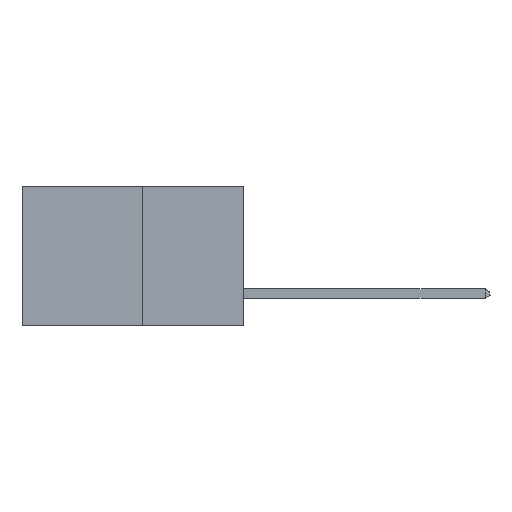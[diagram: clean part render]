
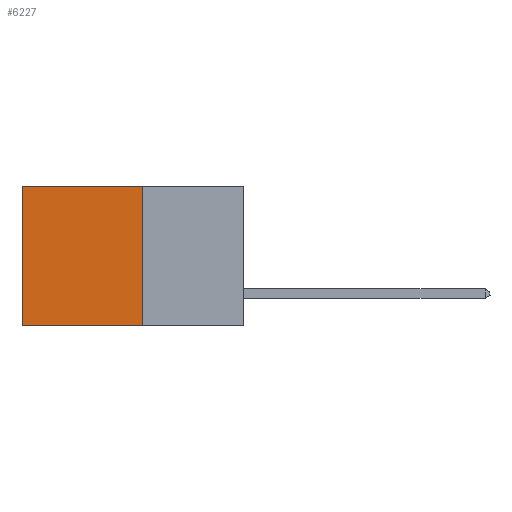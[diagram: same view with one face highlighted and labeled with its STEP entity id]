
A CAD part, left-side view. The second image highlights one B-rep face of the part: STEP entity #6227.
In plain terms, the highlighted planar face has unit normal (-1, 0, 0).
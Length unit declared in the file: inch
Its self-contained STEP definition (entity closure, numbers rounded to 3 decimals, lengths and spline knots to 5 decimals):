
#29 = LINE ( 'NONE', #17643, #5510 ) ;
#1567 = FACE_OUTER_BOUND ( 'NONE', #23449, .T. ) ;
#1588 = ORIENTED_EDGE ( 'NONE', *, *, #8246, .T. ) ;
#4733 = CARTESIAN_POINT ( 'NONE',  ( 0.277, 0.27, 0. ) ) ;
#4839 = CARTESIAN_POINT ( 'NONE',  ( 0.277, 0.59, -0.37 ) ) ;
#5190 = LINE ( 'NONE', #4733, #28686 ) ;
#5510 = VECTOR ( 'NONE', #18485, 39.37008 ) ;
#5772 = DIRECTION ( 'NONE',  ( 0., 1., 0. ) ) ;
#6227 = ADVANCED_FACE ( 'NONE', ( #1567 ), #15031, .F. ) ;
#8246 = EDGE_CURVE ( 'NONE', #19467, #26745, #29, .T. ) ;
#9093 = EDGE_CURVE ( 'NONE', #21050, #10679, #17947, .T. ) ;
#9815 = CARTESIAN_POINT ( 'NONE',  ( 0.277, 0.27, 0. ) ) ;
#10679 = VERTEX_POINT ( 'NONE', #17119 ) ;
#11189 = CARTESIAN_POINT ( 'NONE',  ( 0.277, 0.27, -0.37 ) ) ;
#11669 = VECTOR ( 'NONE', #21087, 39.37008 ) ;
#11834 = LINE ( 'NONE', #11189, #29878 ) ;
#12332 = ORIENTED_EDGE ( 'NONE', *, *, #19632, .F. ) ;
#15031 = PLANE ( 'NONE',  #21664 ) ;
#15071 = DIRECTION ( 'NONE',  ( 0., 0., -1. ) ) ;
#15459 = ORIENTED_EDGE ( 'NONE', *, *, #16561, .T. ) ;
#16561 = EDGE_CURVE ( 'NONE', #21050, #19467, #5190, .T. ) ;
#16855 = ORIENTED_EDGE ( 'NONE', *, *, #9093, .F. ) ;
#17119 = CARTESIAN_POINT ( 'NONE',  ( 0.277, 0.27, -0.37 ) ) ;
#17614 = DIRECTION ( 'NONE',  ( 1., 0., 0. ) ) ;
#17643 = CARTESIAN_POINT ( 'NONE',  ( 0.277, 0.59, -0.37 ) ) ;
#17775 = CARTESIAN_POINT ( 'NONE',  ( 0.277, 0.59, 0. ) ) ;
#17947 = LINE ( 'NONE', #30045, #11669 ) ;
#18485 = DIRECTION ( 'NONE',  ( 0., 0., -1. ) ) ;
#19467 = VERTEX_POINT ( 'NONE', #17775 ) ;
#19632 = EDGE_CURVE ( 'NONE', #10679, #26745, #11834, .T. ) ;
#21050 = VERTEX_POINT ( 'NONE', #9815 ) ;
#21087 = DIRECTION ( 'NONE',  ( 0., 0., -1. ) ) ;
#21664 = AXIS2_PLACEMENT_3D ( 'NONE', #22685, #17614, #15071 ) ;
#22685 = CARTESIAN_POINT ( 'NONE',  ( 0.277, 0.27, -0.37 ) ) ;
#23449 = EDGE_LOOP ( 'NONE', ( #1588, #12332, #16855, #15459 ) ) ;
#26745 = VERTEX_POINT ( 'NONE', #4839 ) ;
#27684 = DIRECTION ( 'NONE',  ( 0., 1., 0. ) ) ;
#28686 = VECTOR ( 'NONE', #5772, 39.37008 ) ;
#29878 = VECTOR ( 'NONE', #27684, 39.37008 ) ;
#30045 = CARTESIAN_POINT ( 'NONE',  ( 0.277, 0.27, -0.37 ) ) ;
